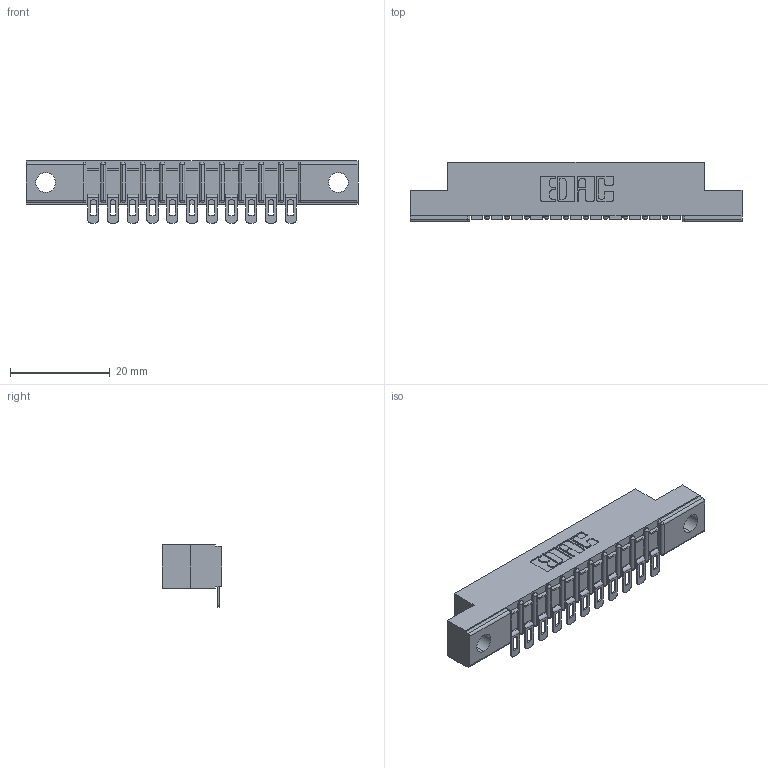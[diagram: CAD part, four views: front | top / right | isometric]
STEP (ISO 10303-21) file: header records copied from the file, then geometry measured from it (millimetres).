
FILE_DESCRIPTION (( 'STEP AP203' ), '1' );
FILE_NAME ('307-011-454-102.STEP', '2020-09-25T10:32:29', ( '' ), ( '' ), 'SwSTEP 2.0', 'SolidWorks 2020', '' );
FILE_SCHEMA (( 'CONFIG_CONTROL_DESIGN' ));
Length unit declared in the file: inch
Products named in the file (3): 307-011-454-102; 307 Part_.128 Dia Mounting Holes; 307-290-002_554
Assembly tree (12 placements, depth 2):
  307-011-454-102
    307 Part_.128 Dia Mounting Holes
    307-290-002_554  x11
Bounding box: 66.6 x 12.01 x 12.52 mm (x, y, z)
Volume: 4307.1 mm3; surface area: 7115.6 mm2
Topology: 12 solids, 12 shells, 1021 faces, 3106 edges, 2036 vertices
Faces by surface type: plane 576, cylinder 421, sphere 24
Entity records: 14219 total; most frequent: CARTESIAN_POINT 2394, ORIENTED_EDGE 2384, DIRECTION 2346, EDGE_CURVE 1192, LINE 890, VECTOR 890, VERTEX_POINT 776, AXIS2_PLACEMENT_3D 728
